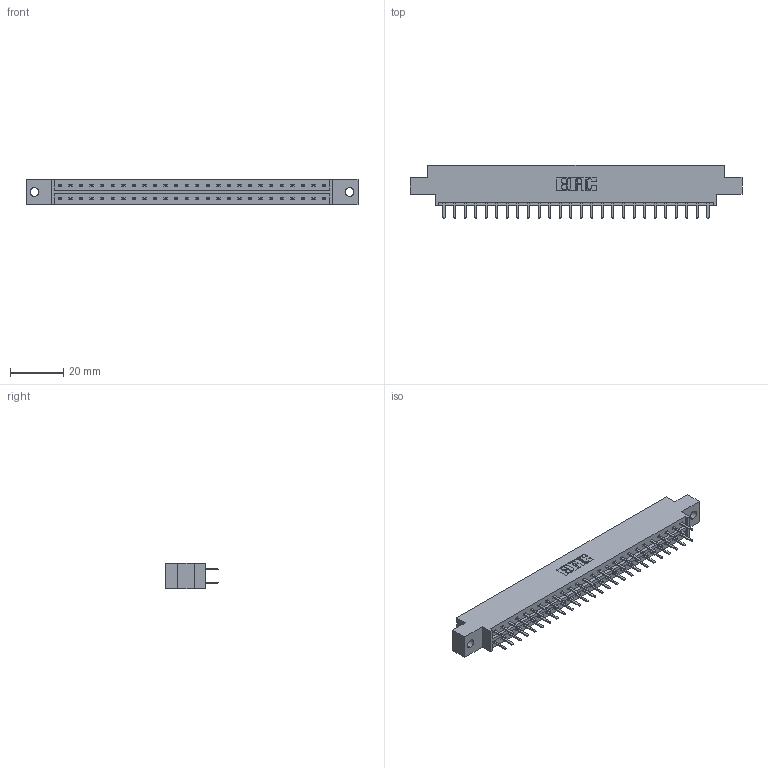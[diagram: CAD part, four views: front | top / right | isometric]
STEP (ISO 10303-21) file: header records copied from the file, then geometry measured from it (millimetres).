
FILE_DESCRIPTION (( 'STEP AP203' ), '1' );
FILE_NAME ('333-052-520-802.STEP', '2018-08-04T01:51:51', ( '' ), ( '' ), 'SwSTEP 2.0', 'SolidWorks 2016', '' );
FILE_SCHEMA (( 'CONFIG_CONTROL_DESIGN' ));
Length unit declared in the file: inch
Products named in the file (3): 333 Part_Offset - .128 Dia; 345-292-001_345-293-120; 333-052-520-802
Assembly tree (53 placements, depth 2):
  333-052-520-802
    333 Part_Offset - .128 Dia
    345-292-001_345-293-120  x52
Bounding box: 124.56 x 20.02 x 9.4 mm (x, y, z)
Volume: 12280.1 mm3; surface area: 14233.1 mm2
Topology: 53 solids, 53 shells, 3030 faces, 8799 edges, 5726 vertices
Faces by surface type: plane 2050, cylinder 980
Entity records: 19045 total; most frequent: CARTESIAN_POINT 3190, ORIENTED_EDGE 3114, DIRECTION 2741, EDGE_CURVE 1557, LINE 1425, VECTOR 1425, VERTEX_POINT 1034, AXIS2_PLACEMENT_3D 658
